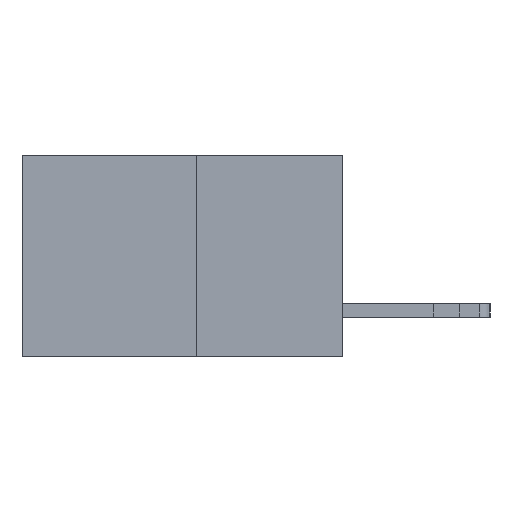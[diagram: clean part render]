
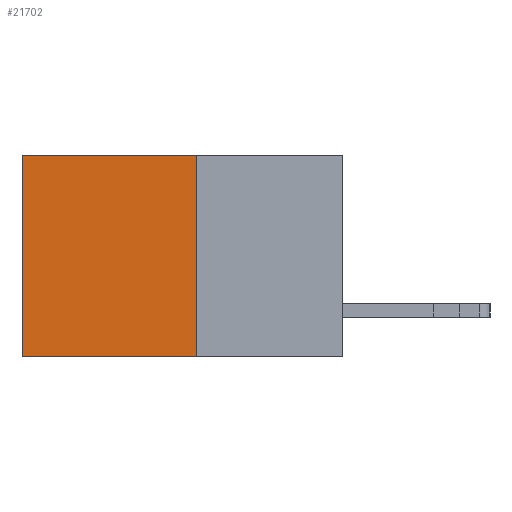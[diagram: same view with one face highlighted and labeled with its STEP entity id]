
A CAD part, left-side view. The second image highlights one B-rep face of the part: STEP entity #21702.
In plain terms, the highlighted planar face has unit normal (-1, 0, 0).
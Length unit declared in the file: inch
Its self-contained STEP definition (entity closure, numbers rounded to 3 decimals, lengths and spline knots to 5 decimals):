
#30 = ORIENTED_EDGE ( 'NONE', *, *, #8464, .T. ) ;
#268 = VECTOR ( 'NONE', #1707, 39.37008 ) ;
#922 = LINE ( 'NONE', #15495, #268 ) ;
#944 = FACE_OUTER_BOUND ( 'NONE', #6174, .T. ) ;
#1707 = DIRECTION ( 'NONE',  ( 0., 0., -1. ) ) ;
#2760 = VECTOR ( 'NONE', #24563, 39.37008 ) ;
#4106 = CARTESIAN_POINT ( 'NONE',  ( 0.277, 0.27, -0.37 ) ) ;
#5240 = EDGE_CURVE ( 'NONE', #8698, #11803, #922, .T. ) ;
#6174 = EDGE_LOOP ( 'NONE', ( #9773, #17049, #12413, #30 ) ) ;
#7657 = LINE ( 'NONE', #9950, #22351 ) ;
#8464 = EDGE_CURVE ( 'NONE', #8698, #22826, #23514, .T. ) ;
#8698 = VERTEX_POINT ( 'NONE', #23400 ) ;
#9773 = ORIENTED_EDGE ( 'NONE', *, *, #16677, .T. ) ;
#9950 = CARTESIAN_POINT ( 'NONE',  ( 0.277, 0.59, -0.37 ) ) ;
#10032 = LINE ( 'NONE', #16410, #19626 ) ;
#11803 = VERTEX_POINT ( 'NONE', #11982 ) ;
#11882 = PLANE ( 'NONE',  #14608 ) ;
#11982 = CARTESIAN_POINT ( 'NONE',  ( 0.277, 0.27, -0.37 ) ) ;
#12047 = DIRECTION ( 'NONE',  ( 0., 0., -1. ) ) ;
#12413 = ORIENTED_EDGE ( 'NONE', *, *, #5240, .F. ) ;
#13426 = CARTESIAN_POINT ( 'NONE',  ( 0.277, 0.59, -0.37 ) ) ;
#14174 = CARTESIAN_POINT ( 'NONE',  ( 0.277, 0.59, 0. ) ) ;
#14608 = AXIS2_PLACEMENT_3D ( 'NONE', #4106, #23580, #12047 ) ;
#14668 = EDGE_CURVE ( 'NONE', #11803, #17786, #10032, .T. ) ;
#14896 = CARTESIAN_POINT ( 'NONE',  ( 0.277, 0.27, 0. ) ) ;
#15495 = CARTESIAN_POINT ( 'NONE',  ( 0.277, 0.27, -0.37 ) ) ;
#16410 = CARTESIAN_POINT ( 'NONE',  ( 0.277, 0.27, -0.37 ) ) ;
#16677 = EDGE_CURVE ( 'NONE', #22826, #17786, #7657, .T. ) ;
#17049 = ORIENTED_EDGE ( 'NONE', *, *, #14668, .F. ) ;
#17786 = VERTEX_POINT ( 'NONE', #13426 ) ;
#19626 = VECTOR ( 'NONE', #22100, 39.37008 ) ;
#21421 = DIRECTION ( 'NONE',  ( 0., 0., -1. ) ) ;
#21702 = ADVANCED_FACE ( 'NONE', ( #944 ), #11882, .F. ) ;
#22100 = DIRECTION ( 'NONE',  ( 0., 1., 0. ) ) ;
#22351 = VECTOR ( 'NONE', #21421, 39.37008 ) ;
#22826 = VERTEX_POINT ( 'NONE', #14174 ) ;
#23400 = CARTESIAN_POINT ( 'NONE',  ( 0.277, 0.27, 0. ) ) ;
#23514 = LINE ( 'NONE', #14896, #2760 ) ;
#23580 = DIRECTION ( 'NONE',  ( 1., 0., 0. ) ) ;
#24563 = DIRECTION ( 'NONE',  ( 0., 1., 0. ) ) ;
